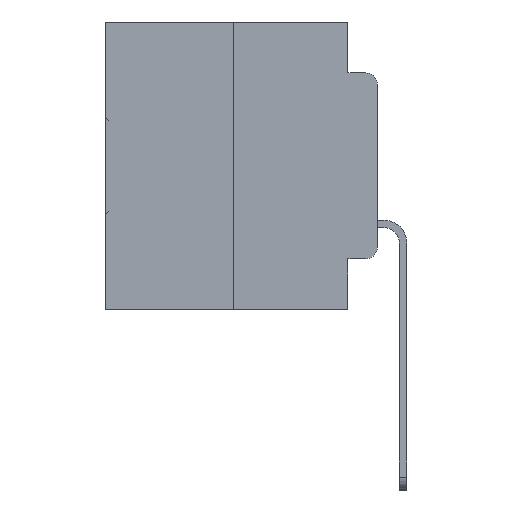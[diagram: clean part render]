
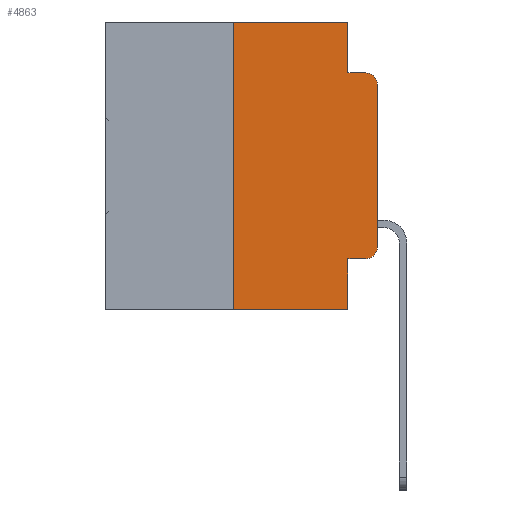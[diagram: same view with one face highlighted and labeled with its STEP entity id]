
A CAD part, left-side view. The second image highlights one B-rep face of the part: STEP entity #4863.
In plain terms, the highlighted planar face has unit normal (-1, 0, 0).
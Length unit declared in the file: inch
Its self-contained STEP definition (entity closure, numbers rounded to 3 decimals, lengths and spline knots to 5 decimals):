
#1 = VERTEX_POINT ( 'NONE', #3423 ) ;
#617 = EDGE_CURVE ( 'NONE', #1308, #26620, #29698, .T. ) ;
#764 = LINE ( 'NONE', #3532, #14591 ) ;
#859 = CARTESIAN_POINT ( 'NONE',  ( 0., 0.051, -0.0885 ) ) ;
#1112 = CARTESIAN_POINT ( 'NONE',  ( 0., 0.051, -0.0885 ) ) ;
#1308 = VERTEX_POINT ( 'NONE', #8464 ) ;
#2062 = VECTOR ( 'NONE', #31100, 39.37008 ) ;
#2782 = VERTEX_POINT ( 'NONE', #30674 ) ;
#3058 = CARTESIAN_POINT ( 'NONE',  ( 0., 0.25, -0.5 ) ) ;
#3083 = DIRECTION ( 'NONE',  ( 0., 0., -1. ) ) ;
#3423 = CARTESIAN_POINT ( 'NONE',  ( 0., 0.051, 0. ) ) ;
#3430 = VECTOR ( 'NONE', #28749, 39.37008 ) ;
#3451 = EDGE_LOOP ( 'NONE', ( #18980, #15510, #17463, #12718, #20530, #22478, #27466, #19328, #14583, #6119 ) ) ;
#3532 = CARTESIAN_POINT ( 'NONE',  ( 0., 0.051, 0. ) ) ;
#4545 = EDGE_CURVE ( 'NONE', #30504, #2782, #23648, .T. ) ;
#4863 = ADVANCED_FACE ( 'NONE', ( #23181 ), #31340, .F. ) ;
#4971 = VERTEX_POINT ( 'NONE', #27069 ) ;
#6119 = ORIENTED_EDGE ( 'NONE', *, *, #15196, .T. ) ;
#7510 = VERTEX_POINT ( 'NONE', #12039 ) ;
#7800 = VERTEX_POINT ( 'NONE', #25872 ) ;
#8464 = CARTESIAN_POINT ( 'NONE',  ( 0., 0., -0.3915 ) ) ;
#8649 = LINE ( 'NONE', #26656, #13102 ) ;
#8987 = CARTESIAN_POINT ( 'NONE',  ( 0., 0.473, 0. ) ) ;
#9108 = DIRECTION ( 'NONE',  ( 0., -1., 0. ) ) ;
#10250 = VECTOR ( 'NONE', #16145, 39.37008 ) ;
#10371 = LINE ( 'NONE', #859, #3430 ) ;
#10928 = CARTESIAN_POINT ( 'NONE',  ( 0., 0.051, 0. ) ) ;
#11376 = DIRECTION ( 'NONE',  ( 0., 0., 1. ) ) ;
#11422 = DIRECTION ( 'NONE',  ( -1., 0., 0. ) ) ;
#12039 = CARTESIAN_POINT ( 'NONE',  ( 0., 0.051, -0.4115 ) ) ;
#12718 = ORIENTED_EDGE ( 'NONE', *, *, #25178, .F. ) ;
#12986 = CARTESIAN_POINT ( 'NONE',  ( 0., 0.02, -0.1085 ) ) ;
#13102 = VECTOR ( 'NONE', #9108, 39.37008 ) ;
#13612 = CIRCLE ( 'NONE', #18625, 0.02 ) ;
#13626 = LINE ( 'NONE', #28773, #19551 ) ;
#14583 = ORIENTED_EDGE ( 'NONE', *, *, #18576, .T. ) ;
#14591 = VECTOR ( 'NONE', #21420, 39.37008 ) ;
#14635 = CIRCLE ( 'NONE', #27084, 0.02 ) ;
#15196 = EDGE_CURVE ( 'NONE', #4971, #1308, #13612, .T. ) ;
#15510 = ORIENTED_EDGE ( 'NONE', *, *, #31705, .T. ) ;
#15561 = DIRECTION ( 'NONE',  ( 0., 0., -1. ) ) ;
#15823 = VECTOR ( 'NONE', #3083, 39.37008 ) ;
#16009 = CARTESIAN_POINT ( 'NONE',  ( 0., 0.473, 0. ) ) ;
#16145 = DIRECTION ( 'NONE',  ( 0., -1., 0. ) ) ;
#16744 = DIRECTION ( 'NONE',  ( 0., 0., -1. ) ) ;
#17203 = VERTEX_POINT ( 'NONE', #1112 ) ;
#17463 = ORIENTED_EDGE ( 'NONE', *, *, #28421, .F. ) ;
#18554 = DIRECTION ( 'NONE',  ( 0., -1., 0. ) ) ;
#18576 = EDGE_CURVE ( 'NONE', #7510, #4971, #8649, .T. ) ;
#18625 = AXIS2_PLACEMENT_3D ( 'NONE', #26387, #11422, #28818 ) ;
#18980 = ORIENTED_EDGE ( 'NONE', *, *, #617, .T. ) ;
#19252 = VERTEX_POINT ( 'NONE', #27252 ) ;
#19328 = ORIENTED_EDGE ( 'NONE', *, *, #20247, .F. ) ;
#19551 = VECTOR ( 'NONE', #11376, 39.37008 ) ;
#20247 = EDGE_CURVE ( 'NONE', #7510, #2782, #22448, .T. ) ;
#20530 = ORIENTED_EDGE ( 'NONE', *, *, #29068, .F. ) ;
#21420 = DIRECTION ( 'NONE',  ( 0., 0., -1. ) ) ;
#22448 = LINE ( 'NONE', #10928, #15823 ) ;
#22478 = ORIENTED_EDGE ( 'NONE', *, *, #23543, .F. ) ;
#23181 = FACE_OUTER_BOUND ( 'NONE', #3451, .T. ) ;
#23543 = EDGE_CURVE ( 'NONE', #30504, #19252, #13626, .T. ) ;
#23550 = CARTESIAN_POINT ( 'NONE',  ( 0., 0.473, -0.5 ) ) ;
#23648 = LINE ( 'NONE', #23550, #10250 ) ;
#23850 = CARTESIAN_POINT ( 'NONE',  ( 0., 0., -0.1085 ) ) ;
#24617 = AXIS2_PLACEMENT_3D ( 'NONE', #8987, #31447, #16744 ) ;
#25178 = EDGE_CURVE ( 'NONE', #1, #17203, #764, .T. ) ;
#25872 = CARTESIAN_POINT ( 'NONE',  ( 0., 0.02, -0.0885 ) ) ;
#26387 = CARTESIAN_POINT ( 'NONE',  ( 0., 0.02, -0.3915 ) ) ;
#26620 = VERTEX_POINT ( 'NONE', #23850 ) ;
#26656 = CARTESIAN_POINT ( 'NONE',  ( 0., 0.051, -0.4115 ) ) ;
#26816 = VECTOR ( 'NONE', #18554, 39.37008 ) ;
#27069 = CARTESIAN_POINT ( 'NONE',  ( 0., 0.02, -0.4115 ) ) ;
#27084 = AXIS2_PLACEMENT_3D ( 'NONE', #12986, #30274, #15561 ) ;
#27252 = CARTESIAN_POINT ( 'NONE',  ( 0., 0.25, 0. ) ) ;
#27466 = ORIENTED_EDGE ( 'NONE', *, *, #4545, .T. ) ;
#27577 = LINE ( 'NONE', #16009, #26816 ) ;
#28421 = EDGE_CURVE ( 'NONE', #17203, #7800, #10371, .T. ) ;
#28749 = DIRECTION ( 'NONE',  ( 0., -1., 0. ) ) ;
#28761 = CARTESIAN_POINT ( 'NONE',  ( 0., 0., 0. ) ) ;
#28773 = CARTESIAN_POINT ( 'NONE',  ( 0., 0.25, 0. ) ) ;
#28818 = DIRECTION ( 'NONE',  ( 0., 0., -1. ) ) ;
#29068 = EDGE_CURVE ( 'NONE', #19252, #1, #27577, .T. ) ;
#29698 = LINE ( 'NONE', #28761, #2062 ) ;
#30274 = DIRECTION ( 'NONE',  ( -1., 0., 0. ) ) ;
#30504 = VERTEX_POINT ( 'NONE', #3058 ) ;
#30674 = CARTESIAN_POINT ( 'NONE',  ( 0., 0.051, -0.5 ) ) ;
#31100 = DIRECTION ( 'NONE',  ( 0., 0., 1. ) ) ;
#31340 = PLANE ( 'NONE',  #24617 ) ;
#31447 = DIRECTION ( 'NONE',  ( 1., 0., 0. ) ) ;
#31705 = EDGE_CURVE ( 'NONE', #26620, #7800, #14635, .T. ) ;
